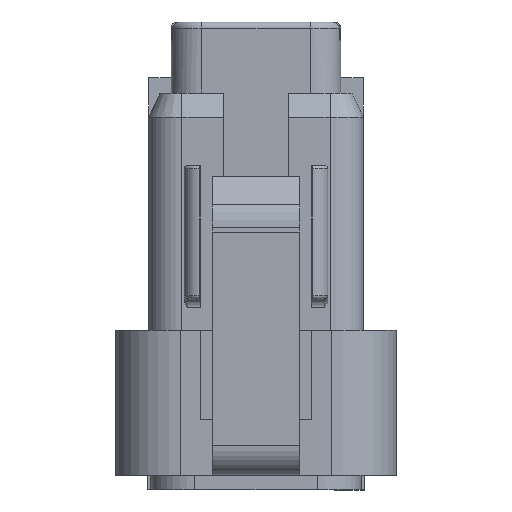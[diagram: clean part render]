
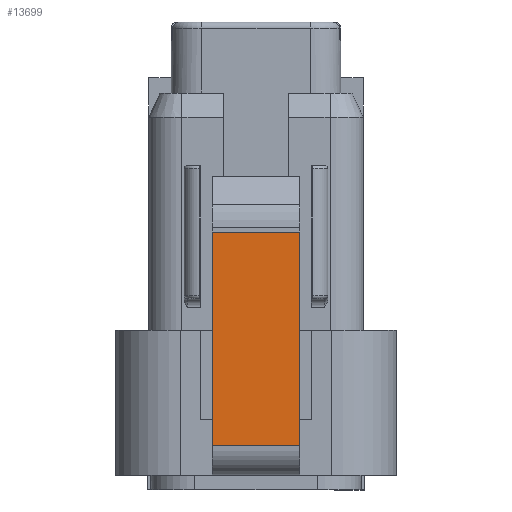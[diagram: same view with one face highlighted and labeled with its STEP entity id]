
A CAD part, front view. The second image highlights one B-rep face of the part: STEP entity #13699.
In plain terms, the highlighted face is planar.
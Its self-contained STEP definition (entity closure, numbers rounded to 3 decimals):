
#194 = CARTESIAN_POINT ( 'NONE',  ( 1.45, 10.25, 5.325 ) ) ;
#222 = ORIENTED_EDGE ( 'NONE', *, *, #10751, .T. ) ;
#540 = LINE ( 'NONE', #10438, #4200 ) ;
#1052 = VECTOR ( 'NONE', #20173, 1000. ) ;
#2095 = FACE_OUTER_BOUND ( 'NONE', #3359, .T. ) ;
#2790 = AXIS2_PLACEMENT_3D ( 'NONE', #6991, #11577, #18246 ) ;
#2843 = CARTESIAN_POINT ( 'NONE',  ( -1.45, 10.25, 5.325 ) ) ;
#3150 = EDGE_CURVE ( 'NONE', #16087, #13374, #540, .T. ) ;
#3350 = ORIENTED_EDGE ( 'NONE', *, *, #11929, .T. ) ;
#3359 = EDGE_LOOP ( 'NONE', ( #222, #20358, #20928, #3350 ) ) ;
#3697 = EDGE_CURVE ( 'NONE', #13374, #14124, #17392, .T. ) ;
#4200 = VECTOR ( 'NONE', #11714, 1000. ) ;
#6559 = LINE ( 'NONE', #194, #15364 ) ;
#6991 = CARTESIAN_POINT ( 'NONE',  ( 1.45, 10.25, 5.325 ) ) ;
#8969 = CARTESIAN_POINT ( 'NONE',  ( 1.45, 10.25, 5.325 ) ) ;
#9100 = PLANE ( 'NONE',  #2790 ) ;
#10429 = CARTESIAN_POINT ( 'NONE',  ( -1.45, 10.25, 5.325 ) ) ;
#10438 = CARTESIAN_POINT ( 'NONE',  ( 1.45, 10.25, 5.325 ) ) ;
#10482 = VERTEX_POINT ( 'NONE', #14351 ) ;
#10751 = EDGE_CURVE ( 'NONE', #10482, #14124, #20065, .T. ) ;
#11577 = DIRECTION ( 'NONE',  ( 0., 0., 1. ) ) ;
#11714 = DIRECTION ( 'NONE',  ( -1., 0., 0. ) ) ;
#11929 = EDGE_CURVE ( 'NONE', #16087, #10482, #6559, .T. ) ;
#12393 = VECTOR ( 'NONE', #15500, 1000. ) ;
#13374 = VERTEX_POINT ( 'NONE', #10429 ) ;
#13699 = ADVANCED_FACE ( 'NONE', ( #2095 ), #9100, .T. ) ;
#13711 = CARTESIAN_POINT ( 'NONE',  ( 1.45, 17.4, 5.325 ) ) ;
#14124 = VERTEX_POINT ( 'NONE', #18301 ) ;
#14351 = CARTESIAN_POINT ( 'NONE',  ( 1.45, 17.4, 5.325 ) ) ;
#15364 = VECTOR ( 'NONE', #16335, 1000. ) ;
#15500 = DIRECTION ( 'NONE',  ( 0., 1., 0. ) ) ;
#16087 = VERTEX_POINT ( 'NONE', #8969 ) ;
#16335 = DIRECTION ( 'NONE',  ( 0., 1., 0. ) ) ;
#17392 = LINE ( 'NONE', #2843, #12393 ) ;
#18246 = DIRECTION ( 'NONE',  ( 0., 1., 0. ) ) ;
#18301 = CARTESIAN_POINT ( 'NONE',  ( -1.45, 17.4, 5.325 ) ) ;
#20065 = LINE ( 'NONE', #13711, #1052 ) ;
#20173 = DIRECTION ( 'NONE',  ( -1., 0., 0. ) ) ;
#20358 = ORIENTED_EDGE ( 'NONE', *, *, #3697, .F. ) ;
#20928 = ORIENTED_EDGE ( 'NONE', *, *, #3150, .F. ) ;
